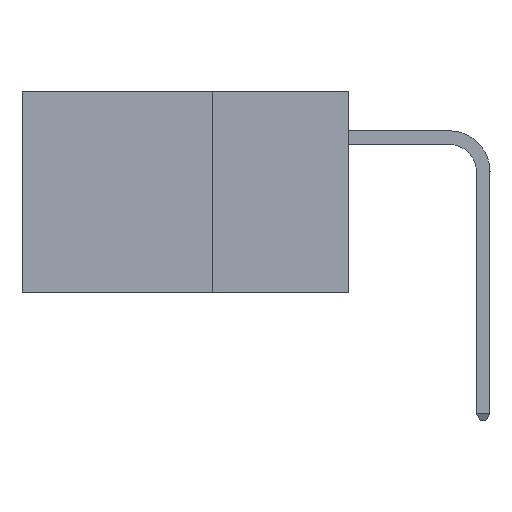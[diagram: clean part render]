
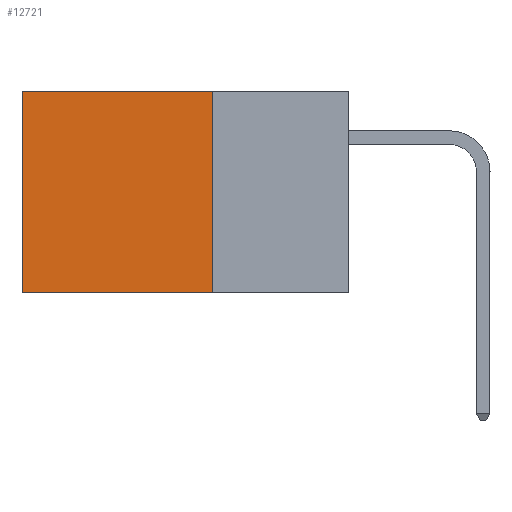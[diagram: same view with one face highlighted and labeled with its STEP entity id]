
A CAD part, left-side view. The second image highlights one B-rep face of the part: STEP entity #12721.
In plain terms, the highlighted planar face has unit normal (-1, 0, 0).
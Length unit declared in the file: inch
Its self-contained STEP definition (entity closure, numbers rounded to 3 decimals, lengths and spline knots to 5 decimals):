
#51 = DIRECTION ( 'NONE',  ( 0., 1., 0. ) ) ;
#329 = LINE ( 'NONE', #17534, #17897 ) ;
#528 = LINE ( 'NONE', #7266, #27799 ) ;
#587 = ORIENTED_EDGE ( 'NONE', *, *, #22483, .F. ) ;
#845 = CARTESIAN_POINT ( 'NONE',  ( 0.2875, 0.25, -0.37 ) ) ;
#1961 = CARTESIAN_POINT ( 'NONE',  ( 0.2875, 0.6, 0. ) ) ;
#2115 = DIRECTION ( 'NONE',  ( 0., 0., -1. ) ) ;
#2665 = ORIENTED_EDGE ( 'NONE', *, *, #22748, .T. ) ;
#4308 = DIRECTION ( 'NONE',  ( 0., 0., -1. ) ) ;
#4445 = VERTEX_POINT ( 'NONE', #845 ) ;
#4598 = FACE_OUTER_BOUND ( 'NONE', #16960, .T. ) ;
#4669 = ORIENTED_EDGE ( 'NONE', *, *, #21502, .T. ) ;
#6404 = EDGE_CURVE ( 'NONE', #4445, #17453, #25430, .T. ) ;
#6495 = PLANE ( 'NONE',  #11410 ) ;
#7050 = DIRECTION ( 'NONE',  ( 0., 1., 0. ) ) ;
#7266 = CARTESIAN_POINT ( 'NONE',  ( 0.2875, 0.25, 0. ) ) ;
#9005 = VECTOR ( 'NONE', #2115, 39.37008 ) ;
#9454 = VERTEX_POINT ( 'NONE', #20837 ) ;
#11410 = AXIS2_PLACEMENT_3D ( 'NONE', #15476, #24437, #4308 ) ;
#11927 = CARTESIAN_POINT ( 'NONE',  ( 0.2875, 0.6, -0.37 ) ) ;
#12721 = ADVANCED_FACE ( 'NONE', ( #4598 ), #6495, .F. ) ;
#14323 = ORIENTED_EDGE ( 'NONE', *, *, #6404, .F. ) ;
#15476 = CARTESIAN_POINT ( 'NONE',  ( 0.2875, 0.25, 0. ) ) ;
#15697 = VERTEX_POINT ( 'NONE', #16594 ) ;
#16594 = CARTESIAN_POINT ( 'NONE',  ( 0.2875, 0.25, 0. ) ) ;
#16686 = VECTOR ( 'NONE', #7050, 39.37008 ) ;
#16960 = EDGE_LOOP ( 'NONE', ( #2665, #14323, #587, #4669 ) ) ;
#17453 = VERTEX_POINT ( 'NONE', #11927 ) ;
#17534 = CARTESIAN_POINT ( 'NONE',  ( 0.2875, 0.25, 0. ) ) ;
#17897 = VECTOR ( 'NONE', #51, 39.37008 ) ;
#19746 = LINE ( 'NONE', #1961, #9005 ) ;
#20837 = CARTESIAN_POINT ( 'NONE',  ( 0.2875, 0.6, 0. ) ) ;
#21502 = EDGE_CURVE ( 'NONE', #15697, #9454, #329, .T. ) ;
#22483 = EDGE_CURVE ( 'NONE', #15697, #4445, #528, .T. ) ;
#22748 = EDGE_CURVE ( 'NONE', #9454, #17453, #19746, .T. ) ;
#24437 = DIRECTION ( 'NONE',  ( 1., 0., 0. ) ) ;
#25430 = LINE ( 'NONE', #27328, #16686 ) ;
#27110 = DIRECTION ( 'NONE',  ( 0., 0., -1. ) ) ;
#27328 = CARTESIAN_POINT ( 'NONE',  ( 0.2875, 0.25, -0.37 ) ) ;
#27799 = VECTOR ( 'NONE', #27110, 39.37008 ) ;
